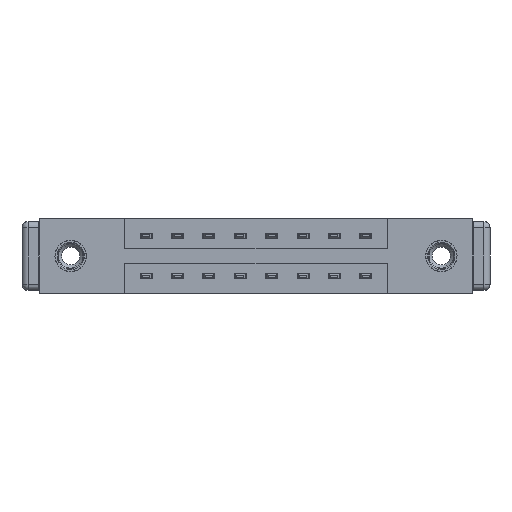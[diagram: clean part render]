
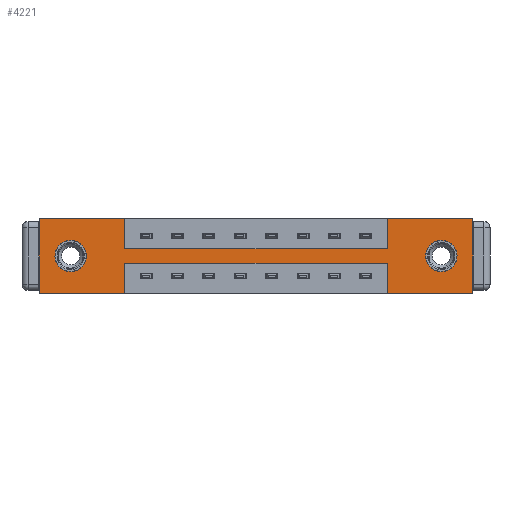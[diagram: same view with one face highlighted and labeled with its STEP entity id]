
A CAD part, front view. The second image highlights one B-rep face of the part: STEP entity #4221.
In plain terms, the highlighted planar face has unit normal (0, -1, 0).
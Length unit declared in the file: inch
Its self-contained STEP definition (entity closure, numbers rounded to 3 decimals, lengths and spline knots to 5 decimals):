
#39 = ORIENTED_EDGE ( 'NONE', *, *, #3450, .T. ) ;
#49 = CARTESIAN_POINT ( 'NONE',  ( 0.155, 0., -0.185 ) ) ;
#67 = VECTOR ( 'NONE', #7832, 39.37008 ) ;
#153 = EDGE_CURVE ( 'NONE', #3214, #12189, #10937, .T. ) ;
#203 = VERTEX_POINT ( 'NONE', #1369 ) ;
#362 = CIRCLE ( 'NONE', #11490, 0.078 ) ;
#549 = EDGE_CURVE ( 'NONE', #8377, #12040, #9812, .T. ) ;
#567 = CARTESIAN_POINT ( 'NONE',  ( 1.729, 0., -0.37 ) ) ;
#583 = CARTESIAN_POINT ( 'NONE',  ( 1.999, 0., -0.185 ) ) ;
#636 = CARTESIAN_POINT ( 'NONE',  ( 2.154, 0., 0. ) ) ;
#689 = ORIENTED_EDGE ( 'NONE', *, *, #4431, .F. ) ;
#771 = EDGE_CURVE ( 'NONE', #203, #4619, #6923, .T. ) ;
#886 = CARTESIAN_POINT ( 'NONE',  ( 0.425, 0., -0.22 ) ) ;
#992 = ORIENTED_EDGE ( 'NONE', *, *, #153, .F. ) ;
#1064 = ORIENTED_EDGE ( 'NONE', *, *, #3908, .F. ) ;
#1331 = VECTOR ( 'NONE', #12270, 39.37008 ) ;
#1369 = CARTESIAN_POINT ( 'NONE',  ( 1.999, 0., -0.263 ) ) ;
#1512 = EDGE_CURVE ( 'NONE', #4619, #203, #362, .T. ) ;
#1586 = DIRECTION ( 'NONE',  ( 0., 0., 1. ) ) ;
#1600 = VERTEX_POINT ( 'NONE', #8261 ) ;
#1655 = ORIENTED_EDGE ( 'NONE', *, *, #1773, .F. ) ;
#1685 = FACE_BOUND ( 'NONE', #9831, .T. ) ;
#1733 = DIRECTION ( 'NONE',  ( 0., 1., 0. ) ) ;
#1773 = EDGE_CURVE ( 'NONE', #12189, #12959, #3828, .T. ) ;
#1812 = ORIENTED_EDGE ( 'NONE', *, *, #3400, .F. ) ;
#1844 = EDGE_CURVE ( 'NONE', #9764, #11634, #8510, .T. ) ;
#2067 = VERTEX_POINT ( 'NONE', #3445 ) ;
#2102 = CARTESIAN_POINT ( 'NONE',  ( 0., 0., 0. ) ) ;
#2340 = AXIS2_PLACEMENT_3D ( 'NONE', #5652, #5569, #4644 ) ;
#2411 = DIRECTION ( 'NONE',  ( -1., 0., 0. ) ) ;
#2580 = DIRECTION ( 'NONE',  ( 0., 0., -1. ) ) ;
#2749 = VECTOR ( 'NONE', #4189, 39.37008 ) ;
#2857 = EDGE_LOOP ( 'NONE', ( #3702, #9449, #1064, #12028, #13036, #2934, #5424, #1655, #992, #689, #1812, #9252 ) ) ;
#2934 = ORIENTED_EDGE ( 'NONE', *, *, #5862, .F. ) ;
#3132 = CARTESIAN_POINT ( 'NONE',  ( 1.999, 0., -0.185 ) ) ;
#3194 = CARTESIAN_POINT ( 'NONE',  ( 0.425, 0., -0.37 ) ) ;
#3214 = VERTEX_POINT ( 'NONE', #4659 ) ;
#3243 = CARTESIAN_POINT ( 'NONE',  ( 0.425, 0., -0.22 ) ) ;
#3397 = CARTESIAN_POINT ( 'NONE',  ( 0., 0., 0. ) ) ;
#3400 = EDGE_CURVE ( 'NONE', #5452, #6749, #6368, .T. ) ;
#3445 = CARTESIAN_POINT ( 'NONE',  ( 1.729, 0., 0. ) ) ;
#3450 = EDGE_CURVE ( 'NONE', #12040, #8377, #7514, .T. ) ;
#3474 = CARTESIAN_POINT ( 'NONE',  ( 0.425, 0., -0.15 ) ) ;
#3702 = ORIENTED_EDGE ( 'NONE', *, *, #8213, .F. ) ;
#3756 = FACE_BOUND ( 'NONE', #9821, .T. ) ;
#3828 = LINE ( 'NONE', #3474, #4333 ) ;
#3908 = EDGE_CURVE ( 'NONE', #11634, #10144, #7657, .T. ) ;
#3957 = CARTESIAN_POINT ( 'NONE',  ( 0.155, 0., -0.185 ) ) ;
#4146 = CARTESIAN_POINT ( 'NONE',  ( 2.154, 0., -0.37 ) ) ;
#4189 = DIRECTION ( 'NONE',  ( -1., 0., 0. ) ) ;
#4221 = ADVANCED_FACE ( 'NONE', ( #3756, #1685, #11923 ), #10702, .T. ) ;
#4262 = LINE ( 'NONE', #2102, #7489 ) ;
#4333 = VECTOR ( 'NONE', #6627, 39.37008 ) ;
#4363 = CARTESIAN_POINT ( 'NONE',  ( 1.729, 0., -0.15 ) ) ;
#4389 = ORIENTED_EDGE ( 'NONE', *, *, #549, .T. ) ;
#4431 = EDGE_CURVE ( 'NONE', #6749, #3214, #4262, .T. ) ;
#4464 = CARTESIAN_POINT ( 'NONE',  ( 1.729, 0., 0. ) ) ;
#4489 = AXIS2_PLACEMENT_3D ( 'NONE', #3957, #11126, #11340 ) ;
#4619 = VERTEX_POINT ( 'NONE', #10661 ) ;
#4644 = DIRECTION ( 'NONE',  ( 0., 0., -1. ) ) ;
#4659 = CARTESIAN_POINT ( 'NONE',  ( 0.425, 0., 0. ) ) ;
#4887 = DIRECTION ( 'NONE',  ( 0., 0., -1. ) ) ;
#5064 = EDGE_CURVE ( 'NONE', #12959, #2067, #8424, .T. ) ;
#5295 = CARTESIAN_POINT ( 'NONE',  ( 0., 0., -0.37 ) ) ;
#5424 = ORIENTED_EDGE ( 'NONE', *, *, #5064, .F. ) ;
#5452 = VERTEX_POINT ( 'NONE', #6848 ) ;
#5569 = DIRECTION ( 'NONE',  ( 0., -1., 0. ) ) ;
#5652 = CARTESIAN_POINT ( 'NONE',  ( 0., 0., -0.37 ) ) ;
#5664 = VERTEX_POINT ( 'NONE', #886 ) ;
#5690 = CARTESIAN_POINT ( 'NONE',  ( 0., 0., 0. ) ) ;
#5862 = EDGE_CURVE ( 'NONE', #2067, #9565, #8727, .T. ) ;
#5986 = VECTOR ( 'NONE', #12557, 39.37008 ) ;
#6368 = LINE ( 'NONE', #5690, #11791 ) ;
#6445 = CARTESIAN_POINT ( 'NONE',  ( 0.155, 0., -0.107 ) ) ;
#6493 = CARTESIAN_POINT ( 'NONE',  ( 0.425, 0., 0. ) ) ;
#6627 = DIRECTION ( 'NONE',  ( 1., 0., 0. ) ) ;
#6749 = VERTEX_POINT ( 'NONE', #13184 ) ;
#6826 = DIRECTION ( 'NONE',  ( 0., 0., -1. ) ) ;
#6848 = CARTESIAN_POINT ( 'NONE',  ( 0., 0., -0.37 ) ) ;
#6923 = CIRCLE ( 'NONE', #8852, 0.078 ) ;
#7161 = VECTOR ( 'NONE', #11297, 39.37008 ) ;
#7489 = VECTOR ( 'NONE', #10351, 39.37008 ) ;
#7514 = CIRCLE ( 'NONE', #4489, 0.078 ) ;
#7582 = CARTESIAN_POINT ( 'NONE',  ( 0., 0., -0.37 ) ) ;
#7657 = LINE ( 'NONE', #9441, #7161 ) ;
#7717 = VECTOR ( 'NONE', #2411, 39.37008 ) ;
#7832 = DIRECTION ( 'NONE',  ( 0., 0., -1. ) ) ;
#7963 = ORIENTED_EDGE ( 'NONE', *, *, #1512, .T. ) ;
#8052 = VECTOR ( 'NONE', #8617, 39.37008 ) ;
#8213 = EDGE_CURVE ( 'NONE', #5664, #1600, #9485, .T. ) ;
#8261 = CARTESIAN_POINT ( 'NONE',  ( 0.425, 0., -0.37 ) ) ;
#8377 = VERTEX_POINT ( 'NONE', #8645 ) ;
#8407 = EDGE_CURVE ( 'NONE', #9565, #9764, #10921, .T. ) ;
#8424 = LINE ( 'NONE', #4464, #10967 ) ;
#8510 = LINE ( 'NONE', #7582, #7717 ) ;
#8617 = DIRECTION ( 'NONE',  ( 0., 0., -1. ) ) ;
#8645 = CARTESIAN_POINT ( 'NONE',  ( 0.155, 0., -0.263 ) ) ;
#8727 = LINE ( 'NONE', #3397, #5986 ) ;
#8777 = EDGE_CURVE ( 'NONE', #1600, #5452, #10758, .T. ) ;
#8852 = AXIS2_PLACEMENT_3D ( 'NONE', #583, #12907, #4887 ) ;
#9252 = ORIENTED_EDGE ( 'NONE', *, *, #8777, .F. ) ;
#9441 = CARTESIAN_POINT ( 'NONE',  ( 1.729, 0., -0.37 ) ) ;
#9449 = ORIENTED_EDGE ( 'NONE', *, *, #9680, .F. ) ;
#9485 = LINE ( 'NONE', #3194, #8052 ) ;
#9522 = AXIS2_PLACEMENT_3D ( 'NONE', #49, #1733, #1586 ) ;
#9565 = VERTEX_POINT ( 'NONE', #11971 ) ;
#9569 = CARTESIAN_POINT ( 'NONE',  ( 0.425, 0., -0.15 ) ) ;
#9680 = EDGE_CURVE ( 'NONE', #10144, #5664, #10762, .T. ) ;
#9713 = ORIENTED_EDGE ( 'NONE', *, *, #771, .T. ) ;
#9764 = VERTEX_POINT ( 'NONE', #4146 ) ;
#9812 = CIRCLE ( 'NONE', #9522, 0.078 ) ;
#9821 = EDGE_LOOP ( 'NONE', ( #7963, #9713 ) ) ;
#9831 = EDGE_LOOP ( 'NONE', ( #39, #4389 ) ) ;
#10144 = VERTEX_POINT ( 'NONE', #11869 ) ;
#10351 = DIRECTION ( 'NONE',  ( 1., 0., 0. ) ) ;
#10661 = CARTESIAN_POINT ( 'NONE',  ( 1.999, 0., -0.107 ) ) ;
#10702 = PLANE ( 'NONE',  #2340 ) ;
#10758 = LINE ( 'NONE', #5295, #1331 ) ;
#10762 = LINE ( 'NONE', #3243, #2749 ) ;
#10921 = LINE ( 'NONE', #636, #11238 ) ;
#10937 = LINE ( 'NONE', #6493, #67 ) ;
#10967 = VECTOR ( 'NONE', #12526, 39.37008 ) ;
#11126 = DIRECTION ( 'NONE',  ( 0., 1., 0. ) ) ;
#11238 = VECTOR ( 'NONE', #6826, 39.37008 ) ;
#11297 = DIRECTION ( 'NONE',  ( 0., 0., 1. ) ) ;
#11340 = DIRECTION ( 'NONE',  ( 0., 0., 1. ) ) ;
#11490 = AXIS2_PLACEMENT_3D ( 'NONE', #3132, #12862, #2580 ) ;
#11634 = VERTEX_POINT ( 'NONE', #567 ) ;
#11791 = VECTOR ( 'NONE', #11881, 39.37008 ) ;
#11869 = CARTESIAN_POINT ( 'NONE',  ( 1.729, 0., -0.22 ) ) ;
#11881 = DIRECTION ( 'NONE',  ( 0., 0., 1. ) ) ;
#11923 = FACE_OUTER_BOUND ( 'NONE', #2857, .T. ) ;
#11971 = CARTESIAN_POINT ( 'NONE',  ( 2.154, 0., 0. ) ) ;
#12028 = ORIENTED_EDGE ( 'NONE', *, *, #1844, .F. ) ;
#12040 = VERTEX_POINT ( 'NONE', #6445 ) ;
#12189 = VERTEX_POINT ( 'NONE', #9569 ) ;
#12270 = DIRECTION ( 'NONE',  ( -1., 0., 0. ) ) ;
#12526 = DIRECTION ( 'NONE',  ( 0., 0., 1. ) ) ;
#12557 = DIRECTION ( 'NONE',  ( 1., 0., 0. ) ) ;
#12862 = DIRECTION ( 'NONE',  ( 0., 1., 0. ) ) ;
#12907 = DIRECTION ( 'NONE',  ( 0., 1., 0. ) ) ;
#12959 = VERTEX_POINT ( 'NONE', #4363 ) ;
#13036 = ORIENTED_EDGE ( 'NONE', *, *, #8407, .F. ) ;
#13184 = CARTESIAN_POINT ( 'NONE',  ( 0., 0., 0. ) ) ;
